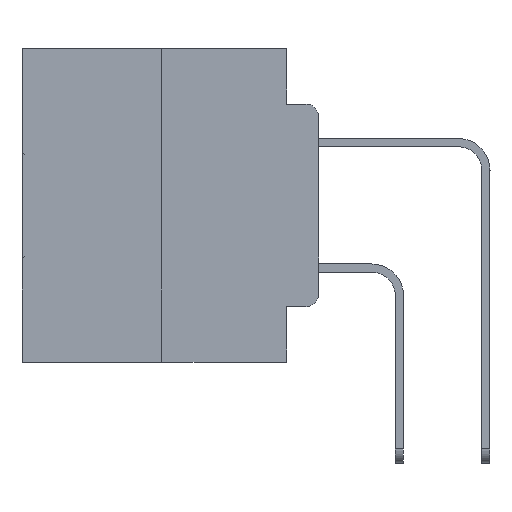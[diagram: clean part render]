
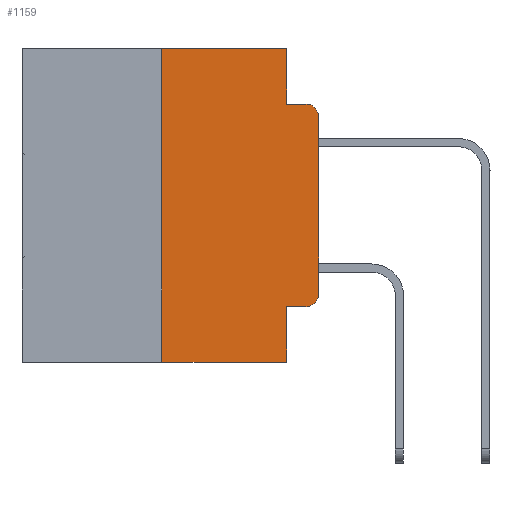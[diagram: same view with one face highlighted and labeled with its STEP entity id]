
A CAD part, left-side view. The second image highlights one B-rep face of the part: STEP entity #1159.
In plain terms, the highlighted planar face has unit normal (-1, 0, 0).
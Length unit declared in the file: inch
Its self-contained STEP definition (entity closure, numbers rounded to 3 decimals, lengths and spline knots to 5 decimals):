
#292 = CARTESIAN_POINT ( 'NONE',  ( 0., 0.051, 0. ) ) ;
#404 = CARTESIAN_POINT ( 'NONE',  ( 0., 0.25, 0. ) ) ;
#511 = DIRECTION ( 'NONE',  ( 0., 0., 1. ) ) ;
#832 = EDGE_CURVE ( 'NONE', #6686, #20668, #17096, .T. ) ;
#873 = ORIENTED_EDGE ( 'NONE', *, *, #17982, .F. ) ;
#875 = ORIENTED_EDGE ( 'NONE', *, *, #7926, .T. ) ;
#1021 = DIRECTION ( 'NONE',  ( 0., 0., -1. ) ) ;
#1159 = ADVANCED_FACE ( 'NONE', ( #19350 ), #24045, .F. ) ;
#1588 = DIRECTION ( 'NONE',  ( 0., 0., -1. ) ) ;
#1822 = EDGE_CURVE ( 'NONE', #4696, #18317, #30318, .T. ) ;
#1962 = CARTESIAN_POINT ( 'NONE',  ( 0., 0.473, 0. ) ) ;
#3139 = ORIENTED_EDGE ( 'NONE', *, *, #12430, .F. ) ;
#3189 = CARTESIAN_POINT ( 'NONE',  ( 0., 0.051, -0.4115 ) ) ;
#3370 = CARTESIAN_POINT ( 'NONE',  ( 0., 0.051, -0.0885 ) ) ;
#3807 = EDGE_CURVE ( 'NONE', #24348, #4840, #19161, .T. ) ;
#3848 = CIRCLE ( 'NONE', #10088, 0.02 ) ;
#4264 = DIRECTION ( 'NONE',  ( 0., 0., -1. ) ) ;
#4423 = EDGE_CURVE ( 'NONE', #20668, #24348, #3848, .T. ) ;
#4696 = VERTEX_POINT ( 'NONE', #14892 ) ;
#4840 = VERTEX_POINT ( 'NONE', #30201 ) ;
#5443 = ORIENTED_EDGE ( 'NONE', *, *, #4423, .T. ) ;
#5972 = VECTOR ( 'NONE', #511, 39.37008 ) ;
#6686 = VERTEX_POINT ( 'NONE', #23636 ) ;
#7476 = LINE ( 'NONE', #1962, #27647 ) ;
#7926 = EDGE_CURVE ( 'NONE', #4840, #22626, #28426, .T. ) ;
#8301 = DIRECTION ( 'NONE',  ( 0., -1., 0. ) ) ;
#8612 = CARTESIAN_POINT ( 'NONE',  ( 0., 0.02, -0.3915 ) ) ;
#9496 = EDGE_LOOP ( 'NONE', ( #28222, #875, #3139, #13876, #30418, #27368, #23356, #873, #27349, #5443 ) ) ;
#9536 = DIRECTION ( 'NONE',  ( 0., -1., 0. ) ) ;
#10088 = AXIS2_PLACEMENT_3D ( 'NONE', #8612, #30785, #1588 ) ;
#10235 = CARTESIAN_POINT ( 'NONE',  ( 0., 0.02, -0.0885 ) ) ;
#11306 = CARTESIAN_POINT ( 'NONE',  ( 0., 0.02, -0.1085 ) ) ;
#11757 = DIRECTION ( 'NONE',  ( 0., -1., 0. ) ) ;
#11764 = CARTESIAN_POINT ( 'NONE',  ( 0., 0.051, -0.0885 ) ) ;
#12208 = AXIS2_PLACEMENT_3D ( 'NONE', #31437, #18878, #4264 ) ;
#12430 = EDGE_CURVE ( 'NONE', #13466, #22626, #28019, .T. ) ;
#12768 = VERTEX_POINT ( 'NONE', #27037 ) ;
#13466 = VERTEX_POINT ( 'NONE', #3370 ) ;
#13876 = ORIENTED_EDGE ( 'NONE', *, *, #26415, .F. ) ;
#13890 = VECTOR ( 'NONE', #23608, 39.37008 ) ;
#14202 = VECTOR ( 'NONE', #15731, 39.37008 ) ;
#14374 = LINE ( 'NONE', #404, #5972 ) ;
#14892 = CARTESIAN_POINT ( 'NONE',  ( 0., 0.25, -0.5 ) ) ;
#15731 = DIRECTION ( 'NONE',  ( 0., 0., 1. ) ) ;
#16276 = VECTOR ( 'NONE', #9536, 39.37008 ) ;
#17096 = LINE ( 'NONE', #3189, #20909 ) ;
#17982 = EDGE_CURVE ( 'NONE', #6686, #18317, #20532, .T. ) ;
#18317 = VERTEX_POINT ( 'NONE', #28808 ) ;
#18878 = DIRECTION ( 'NONE',  ( 1., 0., 0. ) ) ;
#19161 = LINE ( 'NONE', #22728, #14202 ) ;
#19350 = FACE_OUTER_BOUND ( 'NONE', #9496, .T. ) ;
#19368 = EDGE_CURVE ( 'NONE', #4696, #12768, #14374, .T. ) ;
#20532 = LINE ( 'NONE', #27506, #25390 ) ;
#20668 = VERTEX_POINT ( 'NONE', #23236 ) ;
#20909 = VECTOR ( 'NONE', #8301, 39.37008 ) ;
#21193 = CARTESIAN_POINT ( 'NONE',  ( 0., 0.051, 0. ) ) ;
#21511 = DIRECTION ( 'NONE',  ( 0., 0., -1. ) ) ;
#22626 = VERTEX_POINT ( 'NONE', #10235 ) ;
#22728 = CARTESIAN_POINT ( 'NONE',  ( 0., 0., 0. ) ) ;
#22730 = CARTESIAN_POINT ( 'NONE',  ( 0., 0., -0.3915 ) ) ;
#23180 = VERTEX_POINT ( 'NONE', #292 ) ;
#23236 = CARTESIAN_POINT ( 'NONE',  ( 0., 0.02, -0.4115 ) ) ;
#23356 = ORIENTED_EDGE ( 'NONE', *, *, #1822, .T. ) ;
#23608 = DIRECTION ( 'NONE',  ( 0., 0., -1. ) ) ;
#23636 = CARTESIAN_POINT ( 'NONE',  ( 0., 0.051, -0.4115 ) ) ;
#24045 = PLANE ( 'NONE',  #12208 ) ;
#24109 = CARTESIAN_POINT ( 'NONE',  ( 0., 0.473, -0.5 ) ) ;
#24348 = VERTEX_POINT ( 'NONE', #22730 ) ;
#25169 = EDGE_CURVE ( 'NONE', #12768, #23180, #7476, .T. ) ;
#25390 = VECTOR ( 'NONE', #1021, 39.37008 ) ;
#26212 = DIRECTION ( 'NONE',  ( 0., -1., 0. ) ) ;
#26415 = EDGE_CURVE ( 'NONE', #23180, #13466, #26804, .T. ) ;
#26804 = LINE ( 'NONE', #21193, #13890 ) ;
#27037 = CARTESIAN_POINT ( 'NONE',  ( 0., 0.25, 0. ) ) ;
#27349 = ORIENTED_EDGE ( 'NONE', *, *, #832, .T. ) ;
#27368 = ORIENTED_EDGE ( 'NONE', *, *, #19368, .F. ) ;
#27506 = CARTESIAN_POINT ( 'NONE',  ( 0., 0.051, 0. ) ) ;
#27647 = VECTOR ( 'NONE', #11757, 39.37008 ) ;
#27984 = VECTOR ( 'NONE', #26212, 39.37008 ) ;
#28019 = LINE ( 'NONE', #11764, #27984 ) ;
#28163 = AXIS2_PLACEMENT_3D ( 'NONE', #11306, #29054, #21511 ) ;
#28222 = ORIENTED_EDGE ( 'NONE', *, *, #3807, .T. ) ;
#28426 = CIRCLE ( 'NONE', #28163, 0.02 ) ;
#28808 = CARTESIAN_POINT ( 'NONE',  ( 0., 0.051, -0.5 ) ) ;
#29054 = DIRECTION ( 'NONE',  ( -1., 0., 0. ) ) ;
#30201 = CARTESIAN_POINT ( 'NONE',  ( 0., 0., -0.1085 ) ) ;
#30318 = LINE ( 'NONE', #24109, #16276 ) ;
#30418 = ORIENTED_EDGE ( 'NONE', *, *, #25169, .F. ) ;
#30785 = DIRECTION ( 'NONE',  ( -1., 0., 0. ) ) ;
#31437 = CARTESIAN_POINT ( 'NONE',  ( 0., 0.473, 0. ) ) ;
